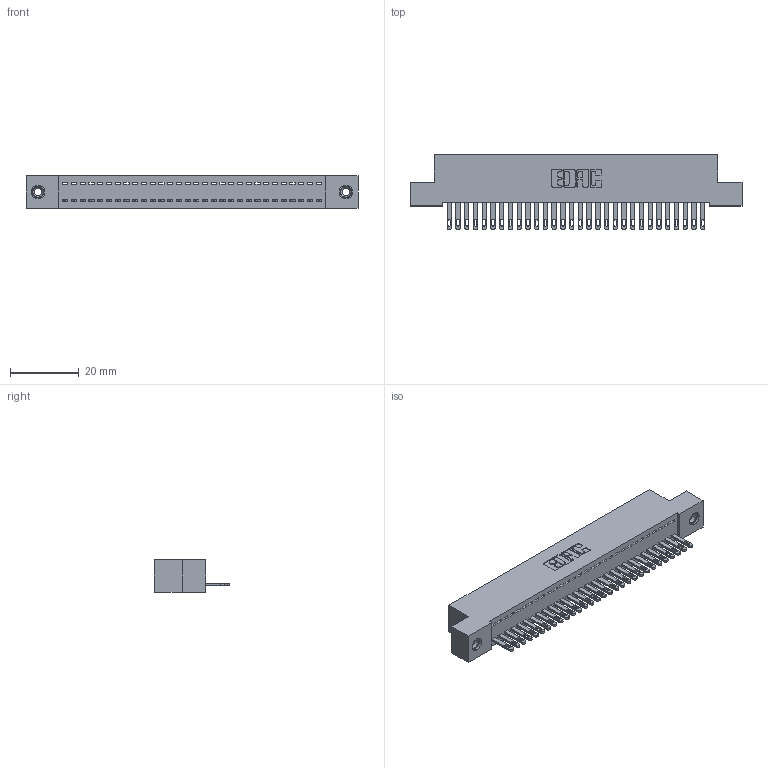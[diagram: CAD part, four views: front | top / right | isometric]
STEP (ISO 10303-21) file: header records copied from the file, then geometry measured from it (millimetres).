
FILE_DESCRIPTION (( 'STEP AP203' ), '1' );
FILE_NAME ('342-030-500-108.STEP', '2018-08-11T15:06:03', ( '' ), ( '' ), 'SwSTEP 2.0', 'SolidWorks 2016', '' );
FILE_SCHEMA (( 'CONFIG_CONTROL_DESIGN' ));
Length unit declared in the file: inch
Products named in the file (4): 345-250-001_345-250-003-102; 342-030-500-108; 342 Part_TI; 345-292-001_345-293-100
Assembly tree (33 placements, depth 2):
  342-030-500-108
    342 Part_TI
    345-292-001_345-293-100  x30
    345-250-001_345-250-003-102  x2
Bounding box: 96.52 x 21.85 x 9.4 mm (x, y, z)
Volume: 8431.6 mm3; surface area: 12234.2 mm2
Topology: 33 solids, 33 shells, 1790 faces, 5475 edges, 3642 vertices
Faces by surface type: plane 1178, cylinder 596, cone 12, torus 4
Entity records: 20876 total; most frequent: CARTESIAN_POINT 3583, ORIENTED_EDGE 3542, DIRECTION 3081, EDGE_CURVE 1771, LINE 1619, VECTOR 1619, VERTEX_POINT 1176, AXIS2_PLACEMENT_3D 731
